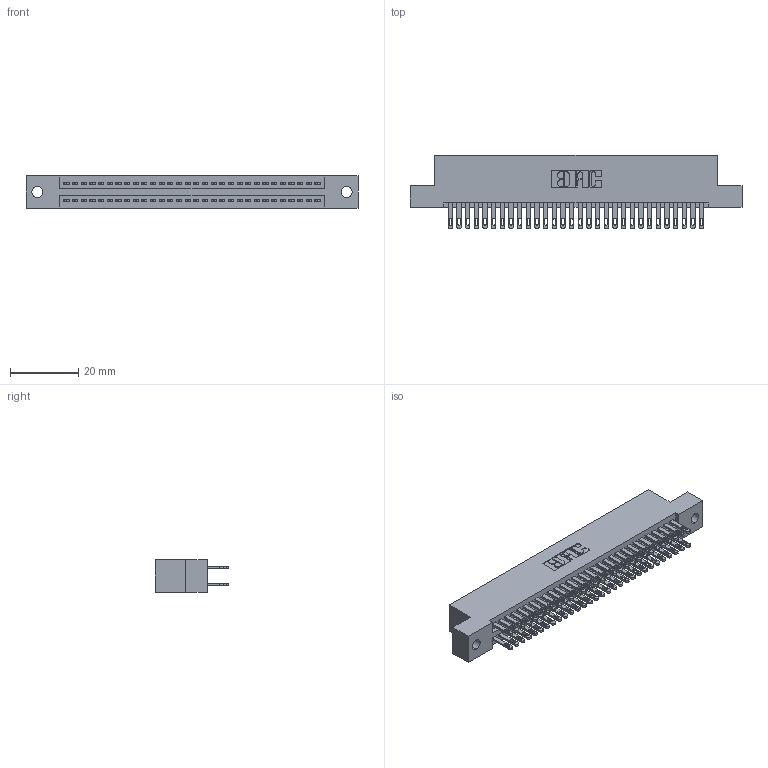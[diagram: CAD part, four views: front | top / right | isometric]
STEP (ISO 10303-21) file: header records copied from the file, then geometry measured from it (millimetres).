
FILE_DESCRIPTION (( 'STEP AP203' ), '1' );
FILE_NAME ('345-060-500-202.STEP', '2018-09-26T22:17:20', ( '' ), ( '' ), 'SwSTEP 2.0', 'SolidWorks 2016', '' );
FILE_SCHEMA (( 'CONFIG_CONTROL_DESIGN' ));
Length unit declared in the file: inch
Products named in the file (3): 345-292-001_345-293-100; 345-060-500-202; 345 Part_Flush Mounting Lugs - 0.128 Dia
Assembly tree (61 placements, depth 2):
  345-060-500-202
    345 Part_Flush Mounting Lugs - 0.128 Dia
    345-292-001_345-293-100  x60
Bounding box: 97.41 x 21.51 x 9.4 mm (x, y, z)
Volume: 9497.7 mm3; surface area: 14146 mm2
Topology: 61 solids, 61 shells, 2886 faces, 8801 edges, 5866 vertices
Faces by surface type: plane 1700, cylinder 1186
Entity records: 25087 total; most frequent: CARTESIAN_POINT 4216, ORIENTED_EDGE 4150, DIRECTION 3735, EDGE_CURVE 2075, LINE 1819, VECTOR 1819, VERTEX_POINT 1382, AXIS2_PLACEMENT_3D 958
